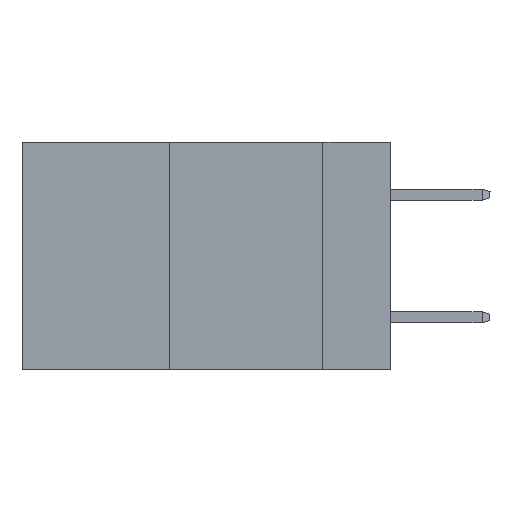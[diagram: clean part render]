
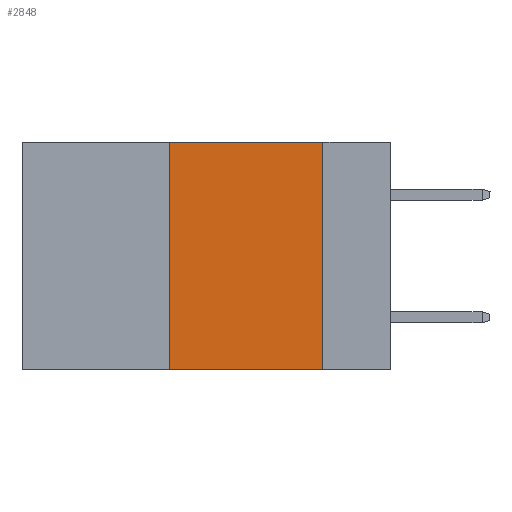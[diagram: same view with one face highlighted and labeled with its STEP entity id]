
A CAD part, left-side view. The second image highlights one B-rep face of the part: STEP entity #2848.
In plain terms, the highlighted planar face has unit normal (-1, 0, 0).
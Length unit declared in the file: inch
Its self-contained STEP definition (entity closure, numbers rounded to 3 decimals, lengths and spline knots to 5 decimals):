
#255 = VERTEX_POINT ( 'NONE', #655 ) ;
#584 = AXIS2_PLACEMENT_3D ( 'NONE', #19174, #19726, #19632 ) ;
#655 = CARTESIAN_POINT ( 'NONE',  ( 0., 0.11, 0. ) ) ;
#1097 = EDGE_CURVE ( 'NONE', #12975, #11170, #13763, .T. ) ;
#1830 = EDGE_CURVE ( 'NONE', #12744, #255, #21479, .T. ) ;
#2363 = CARTESIAN_POINT ( 'NONE',  ( 0., 0.36, -0.37 ) ) ;
#2848 = ADVANCED_FACE ( 'NONE', ( #10281 ), #6613, .F. ) ;
#3031 = ORIENTED_EDGE ( 'NONE', *, *, #16032, .F. ) ;
#3715 = LINE ( 'NONE', #17219, #21598 ) ;
#5983 = LINE ( 'NONE', #9053, #25897 ) ;
#6613 = PLANE ( 'NONE',  #584 ) ;
#6643 = VECTOR ( 'NONE', #24488, 39.37008 ) ;
#7013 = VECTOR ( 'NONE', #19593, 39.37008 ) ;
#7517 = ORIENTED_EDGE ( 'NONE', *, *, #1830, .F. ) ;
#9053 = CARTESIAN_POINT ( 'NONE',  ( 0., 0.11, 0. ) ) ;
#9191 = CARTESIAN_POINT ( 'NONE',  ( 0., 0.6, 0. ) ) ;
#10281 = FACE_OUTER_BOUND ( 'NONE', #23187, .T. ) ;
#11170 = VERTEX_POINT ( 'NONE', #20612 ) ;
#12207 = ORIENTED_EDGE ( 'NONE', *, *, #27027, .F. ) ;
#12744 = VERTEX_POINT ( 'NONE', #27521 ) ;
#12975 = VERTEX_POINT ( 'NONE', #2363 ) ;
#13763 = LINE ( 'NONE', #17699, #7013 ) ;
#16032 = EDGE_CURVE ( 'NONE', #12975, #12744, #3715, .T. ) ;
#17219 = CARTESIAN_POINT ( 'NONE',  ( 0., 0.36, 0. ) ) ;
#17699 = CARTESIAN_POINT ( 'NONE',  ( 0., 0.6, -0.37 ) ) ;
#19174 = CARTESIAN_POINT ( 'NONE',  ( 0., 0.6, 0. ) ) ;
#19593 = DIRECTION ( 'NONE',  ( 0., -1., 0. ) ) ;
#19632 = DIRECTION ( 'NONE',  ( 0., 0., -1. ) ) ;
#19726 = DIRECTION ( 'NONE',  ( 1., 0., 0. ) ) ;
#19989 = ORIENTED_EDGE ( 'NONE', *, *, #1097, .T. ) ;
#20612 = CARTESIAN_POINT ( 'NONE',  ( 0., 0.11, -0.37 ) ) ;
#21479 = LINE ( 'NONE', #9191, #6643 ) ;
#21598 = VECTOR ( 'NONE', #25888, 39.37008 ) ;
#23187 = EDGE_LOOP ( 'NONE', ( #12207, #7517, #3031, #19989 ) ) ;
#24148 = DIRECTION ( 'NONE',  ( 0., 0., -1. ) ) ;
#24488 = DIRECTION ( 'NONE',  ( 0., -1., 0. ) ) ;
#25888 = DIRECTION ( 'NONE',  ( 0., 0., 1. ) ) ;
#25897 = VECTOR ( 'NONE', #24148, 39.37008 ) ;
#27027 = EDGE_CURVE ( 'NONE', #255, #11170, #5983, .T. ) ;
#27521 = CARTESIAN_POINT ( 'NONE',  ( 0., 0.36, 0. ) ) ;
